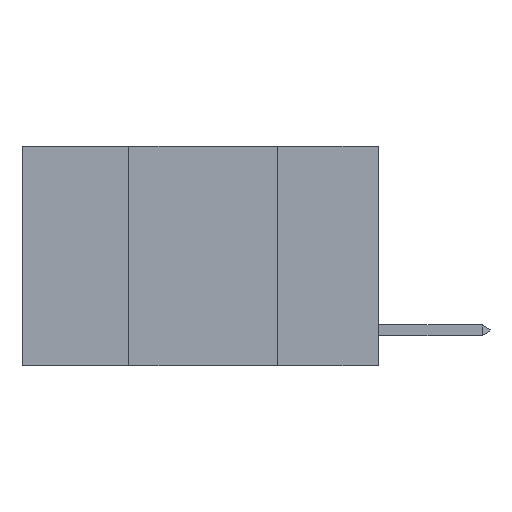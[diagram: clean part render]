
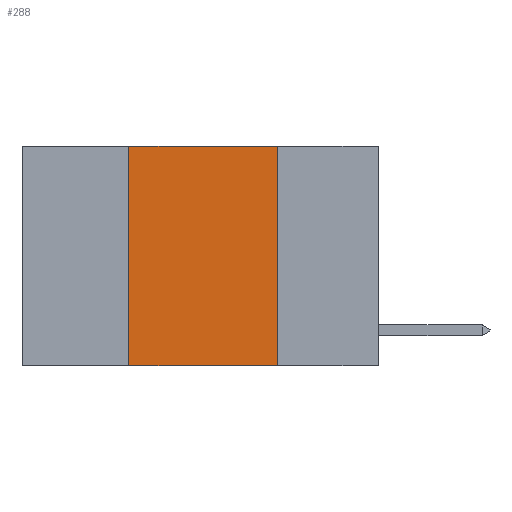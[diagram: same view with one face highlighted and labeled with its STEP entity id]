
A CAD part, left-side view. The second image highlights one B-rep face of the part: STEP entity #288.
In plain terms, the highlighted planar face has unit normal (-1, 0, 0).
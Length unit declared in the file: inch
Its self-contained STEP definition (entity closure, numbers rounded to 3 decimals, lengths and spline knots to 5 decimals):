
#252 = DIRECTION ( 'NONE',  ( 0., 0., -1. ) ) ;
#288 = ADVANCED_FACE ( 'NONE', ( #15815 ), #2821, .F. ) ;
#712 = VERTEX_POINT ( 'NONE', #3985 ) ;
#1417 = ORIENTED_EDGE ( 'NONE', *, *, #20652, .F. ) ;
#1640 = ORIENTED_EDGE ( 'NONE', *, *, #18437, .T. ) ;
#2821 = PLANE ( 'NONE',  #16915 ) ;
#3985 = CARTESIAN_POINT ( 'NONE',  ( 0., 0.17, 0. ) ) ;
#5410 = CARTESIAN_POINT ( 'NONE',  ( 0., 0.6, 0. ) ) ;
#5458 = VECTOR ( 'NONE', #17348, 39.37008 ) ;
#5793 = VECTOR ( 'NONE', #7481, 39.37008 ) ;
#6549 = LINE ( 'NONE', #7296, #5458 ) ;
#7052 = CARTESIAN_POINT ( 'NONE',  ( 0., 0.42, -0.37 ) ) ;
#7125 = DIRECTION ( 'NONE',  ( 0., -1., 0. ) ) ;
#7296 = CARTESIAN_POINT ( 'NONE',  ( 0., 0.42, 0. ) ) ;
#7481 = DIRECTION ( 'NONE',  ( 0., -1., 0. ) ) ;
#10154 = DIRECTION ( 'NONE',  ( 1., 0., 0. ) ) ;
#10413 = ORIENTED_EDGE ( 'NONE', *, *, #20127, .F. ) ;
#10425 = VECTOR ( 'NONE', #13439, 39.37008 ) ;
#11405 = ORIENTED_EDGE ( 'NONE', *, *, #19559, .F. ) ;
#12427 = VERTEX_POINT ( 'NONE', #20600 ) ;
#12485 = VERTEX_POINT ( 'NONE', #19229 ) ;
#13439 = DIRECTION ( 'NONE',  ( 0., 0., -1. ) ) ;
#13554 = LINE ( 'NONE', #5410, #17459 ) ;
#14579 = CARTESIAN_POINT ( 'NONE',  ( 0., 0.6, 0. ) ) ;
#14813 = LINE ( 'NONE', #15102, #10425 ) ;
#15102 = CARTESIAN_POINT ( 'NONE',  ( 0., 0.17, 0. ) ) ;
#15646 = EDGE_LOOP ( 'NONE', ( #1417, #10413, #11405, #1640 ) ) ;
#15815 = FACE_OUTER_BOUND ( 'NONE', #15646, .T. ) ;
#16915 = AXIS2_PLACEMENT_3D ( 'NONE', #14579, #10154, #252 ) ;
#17348 = DIRECTION ( 'NONE',  ( 0., 0., 1. ) ) ;
#17390 = CARTESIAN_POINT ( 'NONE',  ( 0., 0.6, -0.37 ) ) ;
#17459 = VECTOR ( 'NONE', #7125, 39.37008 ) ;
#18437 = EDGE_CURVE ( 'NONE', #21383, #12485, #19083, .T. ) ;
#19083 = LINE ( 'NONE', #17390, #5793 ) ;
#19229 = CARTESIAN_POINT ( 'NONE',  ( 0., 0.17, -0.37 ) ) ;
#19559 = EDGE_CURVE ( 'NONE', #21383, #12427, #6549, .T. ) ;
#20127 = EDGE_CURVE ( 'NONE', #12427, #712, #13554, .T. ) ;
#20600 = CARTESIAN_POINT ( 'NONE',  ( 0., 0.42, 0. ) ) ;
#20652 = EDGE_CURVE ( 'NONE', #712, #12485, #14813, .T. ) ;
#21383 = VERTEX_POINT ( 'NONE', #7052 ) ;
